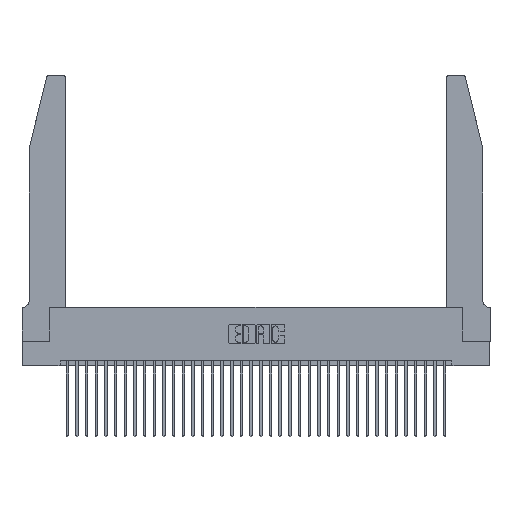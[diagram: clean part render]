
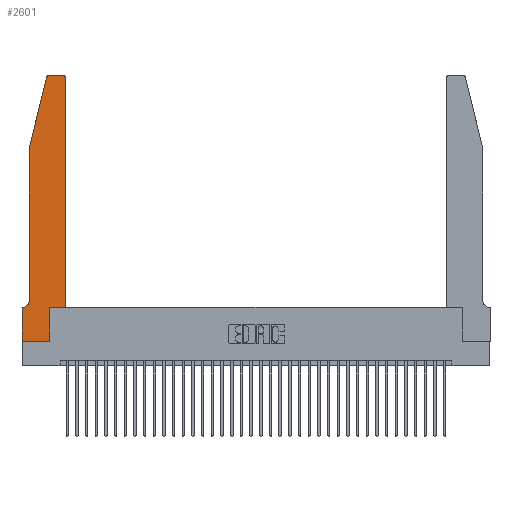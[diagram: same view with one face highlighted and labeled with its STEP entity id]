
A CAD part, top view. The second image highlights one B-rep face of the part: STEP entity #2601.
In plain terms, the highlighted planar face has unit normal (0, 0, 1).
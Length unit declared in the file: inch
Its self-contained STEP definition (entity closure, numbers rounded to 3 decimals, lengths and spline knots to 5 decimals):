
#341 = EDGE_CURVE ( 'NONE', #25035, #6867, #34419, .T. ) ;
#1014 = VERTEX_POINT ( 'NONE', #3525 ) ;
#1229 = EDGE_CURVE ( 'NONE', #28373, #15798, #30510, .T. ) ;
#1368 = ORIENTED_EDGE ( 'NONE', *, *, #15275, .T. ) ;
#1695 = DIRECTION ( 'NONE',  ( -1., 0., 0. ) ) ;
#1699 = LINE ( 'NONE', #8081, #22618 ) ;
#1941 = ORIENTED_EDGE ( 'NONE', *, *, #30631, .T. ) ;
#2274 = DIRECTION ( 'NONE',  ( 0., -1., 0. ) ) ;
#2601 = ADVANCED_FACE ( 'NONE', ( #3975 ), #22171, .T. ) ;
#2621 = ORIENTED_EDGE ( 'NONE', *, *, #10735, .T. ) ;
#2826 = ORIENTED_EDGE ( 'NONE', *, *, #21409, .T. ) ;
#3448 = CARTESIAN_POINT ( 'NONE',  ( 0.4505, 0.35, 0.37 ) ) ;
#3525 = CARTESIAN_POINT ( 'NONE',  ( 0., 0.35, 0.37 ) ) ;
#3672 = CARTESIAN_POINT ( 'NONE',  ( 0.0755, 2., 0.37 ) ) ;
#3975 = FACE_OUTER_BOUND ( 'NONE', #27366, .T. ) ;
#5432 = CARTESIAN_POINT ( 'NONE',  ( 0.284, 2.75, 0.37 ) ) ;
#5703 = ORIENTED_EDGE ( 'NONE', *, *, #26601, .T. ) ;
#6488 = CARTESIAN_POINT ( 'NONE',  ( 0.0755, 0.42, 0.37 ) ) ;
#6502 = EDGE_CURVE ( 'NONE', #15798, #16036, #11569, .T. ) ;
#6821 = LINE ( 'NONE', #23545, #13509 ) ;
#6867 = VERTEX_POINT ( 'NONE', #16647 ) ;
#7195 = DIRECTION ( 'NONE',  ( 1., 0., 0. ) ) ;
#7521 = AXIS2_PLACEMENT_3D ( 'NONE', #27390, #10564, #30151 ) ;
#7675 = CARTESIAN_POINT ( 'NONE',  ( 0.4505, 2.72, 0.37 ) ) ;
#7919 = DIRECTION ( 'NONE',  ( 0., 0., 1. ) ) ;
#8081 = CARTESIAN_POINT ( 'NONE',  ( 0., 0., 0.37 ) ) ;
#8095 = DIRECTION ( 'NONE',  ( 1., 0., 0. ) ) ;
#8139 = VECTOR ( 'NONE', #12880, 39.37008 ) ;
#8247 = VERTEX_POINT ( 'NONE', #31240 ) ;
#8944 = LINE ( 'NONE', #19278, #30452 ) ;
#9049 = CARTESIAN_POINT ( 'NONE',  ( 0.0755, 2., 0.37 ) ) ;
#9205 = VECTOR ( 'NONE', #34222, 39.37008 ) ;
#9209 = EDGE_CURVE ( 'NONE', #16664, #25120, #34951, .T. ) ;
#10272 = CARTESIAN_POINT ( 'NONE',  ( 0.0755, 0.35, 0.37 ) ) ;
#10379 = VERTEX_POINT ( 'NONE', #28326 ) ;
#10564 = DIRECTION ( 'NONE',  ( 0., 0., -1. ) ) ;
#10735 = EDGE_CURVE ( 'NONE', #10379, #1014, #24950, .T. ) ;
#10825 = CARTESIAN_POINT ( 'NONE',  ( 0., 0.35, 0.37 ) ) ;
#11569 = LINE ( 'NONE', #3448, #26499 ) ;
#11648 = VECTOR ( 'NONE', #14516, 39.37008 ) ;
#12525 = LINE ( 'NONE', #22871, #11648 ) ;
#12880 = DIRECTION ( 'NONE',  ( 0., 1., 0. ) ) ;
#12919 = DIRECTION ( 'NONE',  ( 1., 0., 0. ) ) ;
#13509 = VECTOR ( 'NONE', #26343, 39.37008 ) ;
#14516 = DIRECTION ( 'NONE',  ( -1., 0., 0. ) ) ;
#14562 = CARTESIAN_POINT ( 'NONE',  ( 0.4205, 2.72, 0.37 ) ) ;
#14751 = DIRECTION ( 'NONE',  ( 0., 0., 1. ) ) ;
#15266 = ORIENTED_EDGE ( 'NONE', *, *, #23141, .T. ) ;
#15275 = EDGE_CURVE ( 'NONE', #18333, #31567, #25072, .T. ) ;
#15602 = ORIENTED_EDGE ( 'NONE', *, *, #341, .T. ) ;
#15798 = VERTEX_POINT ( 'NONE', #29104 ) ;
#16036 = VERTEX_POINT ( 'NONE', #27662 ) ;
#16647 = CARTESIAN_POINT ( 'NONE',  ( 0.4205, 2.75, 0.37 ) ) ;
#16664 = VERTEX_POINT ( 'NONE', #5432 ) ;
#16941 = ORIENTED_EDGE ( 'NONE', *, *, #9209, .T. ) ;
#18333 = VERTEX_POINT ( 'NONE', #3672 ) ;
#19278 = CARTESIAN_POINT ( 'NONE',  ( 0.0755, 2., 0.37 ) ) ;
#20485 = DIRECTION ( 'NONE',  ( 1., 0., 0. ) ) ;
#21409 = EDGE_CURVE ( 'NONE', #16036, #25035, #6821, .T. ) ;
#22065 = DIRECTION ( 'NONE',  ( -0.239, -0.971, 0. ) ) ;
#22171 = PLANE ( 'NONE',  #30361 ) ;
#22547 = VECTOR ( 'NONE', #7195, 39.37008 ) ;
#22618 = VECTOR ( 'NONE', #2274, 39.37008 ) ;
#22787 = CIRCLE ( 'NONE', #7521, 0.07 ) ;
#22871 = CARTESIAN_POINT ( 'NONE',  ( 0.2605, 2.75, 0.37 ) ) ;
#22973 = ORIENTED_EDGE ( 'NONE', *, *, #28086, .T. ) ;
#23141 = EDGE_CURVE ( 'NONE', #1014, #8247, #1699, .T. ) ;
#23341 = AXIS2_PLACEMENT_3D ( 'NONE', #14562, #14751, #12919 ) ;
#23545 = CARTESIAN_POINT ( 'NONE',  ( 0.4505, 0.35, 0.37 ) ) ;
#24062 = CARTESIAN_POINT ( 'NONE',  ( 0.2865, 0.35, 0.37 ) ) ;
#24278 = LINE ( 'NONE', #34817, #22547 ) ;
#24788 = CARTESIAN_POINT ( 'NONE',  ( 0.284, 2.72, 0.37 ) ) ;
#24950 = LINE ( 'NONE', #10272, #31416 ) ;
#24962 = DIRECTION ( 'NONE',  ( 0., 0., 1. ) ) ;
#25035 = VERTEX_POINT ( 'NONE', #7675 ) ;
#25072 = LINE ( 'NONE', #9049, #9205 ) ;
#25120 = VERTEX_POINT ( 'NONE', #35980 ) ;
#26343 = DIRECTION ( 'NONE',  ( 0., 1., 0. ) ) ;
#26499 = VECTOR ( 'NONE', #20485, 39.37008 ) ;
#26601 = EDGE_CURVE ( 'NONE', #6867, #16664, #12525, .T. ) ;
#27366 = EDGE_LOOP ( 'NONE', ( #5703, #16941, #32142, #1368, #1941, #2621, #15266, #22973, #29310, #32181, #2826, #15602 ) ) ;
#27390 = CARTESIAN_POINT ( 'NONE',  ( 0.0055, 0.42, 0.37 ) ) ;
#27584 = DIRECTION ( 'NONE',  ( 1., 0., 0. ) ) ;
#27662 = CARTESIAN_POINT ( 'NONE',  ( 0.4505, 0.35, 0.37 ) ) ;
#28086 = EDGE_CURVE ( 'NONE', #8247, #28373, #24278, .T. ) ;
#28326 = CARTESIAN_POINT ( 'NONE',  ( 0.0055, 0.35, 0.37 ) ) ;
#28373 = VERTEX_POINT ( 'NONE', #33501 ) ;
#29104 = CARTESIAN_POINT ( 'NONE',  ( 0.2865, 0.35, 0.37 ) ) ;
#29310 = ORIENTED_EDGE ( 'NONE', *, *, #1229, .T. ) ;
#30151 = DIRECTION ( 'NONE',  ( -1., 0., 0. ) ) ;
#30361 = AXIS2_PLACEMENT_3D ( 'NONE', #10825, #24962, #8095 ) ;
#30452 = VECTOR ( 'NONE', #22065, 39.37008 ) ;
#30510 = LINE ( 'NONE', #24062, #8139 ) ;
#30631 = EDGE_CURVE ( 'NONE', #31567, #10379, #22787, .T. ) ;
#31240 = CARTESIAN_POINT ( 'NONE',  ( 0., 0., 0.37 ) ) ;
#31416 = VECTOR ( 'NONE', #1695, 39.37008 ) ;
#31567 = VERTEX_POINT ( 'NONE', #6488 ) ;
#31975 = EDGE_CURVE ( 'NONE', #25120, #18333, #8944, .T. ) ;
#32142 = ORIENTED_EDGE ( 'NONE', *, *, #31975, .T. ) ;
#32181 = ORIENTED_EDGE ( 'NONE', *, *, #6502, .T. ) ;
#33501 = CARTESIAN_POINT ( 'NONE',  ( 0.2865, 0., 0.37 ) ) ;
#34222 = DIRECTION ( 'NONE',  ( 0., -1., 0. ) ) ;
#34419 = CIRCLE ( 'NONE', #23341, 0.03 ) ;
#34817 = CARTESIAN_POINT ( 'NONE',  ( 0., 0., 0.37 ) ) ;
#34951 = CIRCLE ( 'NONE', #35067, 0.03 ) ;
#35067 = AXIS2_PLACEMENT_3D ( 'NONE', #24788, #7919, #27584 ) ;
#35980 = CARTESIAN_POINT ( 'NONE',  ( 0.25487, 2.72718, 0.37 ) ) ;
